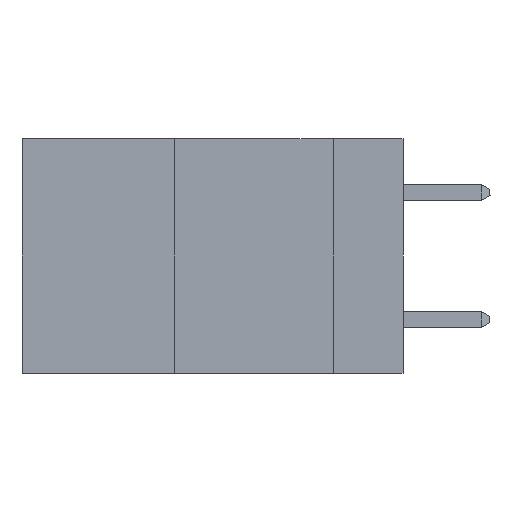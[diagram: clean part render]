
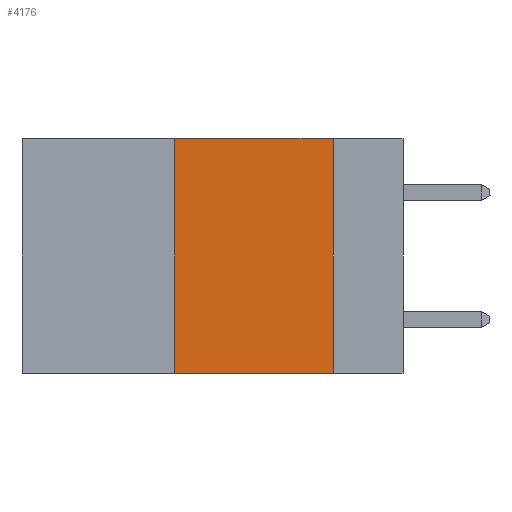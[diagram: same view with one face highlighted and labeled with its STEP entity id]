
A CAD part, left-side view. The second image highlights one B-rep face of the part: STEP entity #4176.
In plain terms, the highlighted planar face has unit normal (-1, 0, 0).
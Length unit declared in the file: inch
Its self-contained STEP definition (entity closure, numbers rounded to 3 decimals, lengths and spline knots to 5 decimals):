
#169 = CARTESIAN_POINT ( 'NONE',  ( 0., 0.36, 0. ) ) ;
#264 = DIRECTION ( 'NONE',  ( 1., 0., 0. ) ) ;
#759 = ORIENTED_EDGE ( 'NONE', *, *, #2254, .F. ) ;
#1437 = EDGE_CURVE ( 'NONE', #4268, #16691, #3382, .T. ) ;
#2254 = EDGE_CURVE ( 'NONE', #16691, #3262, #9374, .T. ) ;
#2404 = CARTESIAN_POINT ( 'NONE',  ( 0., 0.6, 0. ) ) ;
#2499 = EDGE_CURVE ( 'NONE', #23659, #3262, #10859, .T. ) ;
#2549 = ORIENTED_EDGE ( 'NONE', *, *, #15353, .F. ) ;
#2704 = ORIENTED_EDGE ( 'NONE', *, *, #1437, .F. ) ;
#3262 = VERTEX_POINT ( 'NONE', #7851 ) ;
#3382 = LINE ( 'NONE', #11134, #20433 ) ;
#3867 = LINE ( 'NONE', #169, #15531 ) ;
#4100 = CARTESIAN_POINT ( 'NONE',  ( 0., 0.11, 0. ) ) ;
#4176 = ADVANCED_FACE ( 'NONE', ( #7513 ), #15871, .F. ) ;
#4268 = VERTEX_POINT ( 'NONE', #10286 ) ;
#5139 = DIRECTION ( 'NONE',  ( 0., -1., 0. ) ) ;
#7050 = CARTESIAN_POINT ( 'NONE',  ( 0., 0.6, -0.37 ) ) ;
#7513 = FACE_OUTER_BOUND ( 'NONE', #17952, .T. ) ;
#7851 = CARTESIAN_POINT ( 'NONE',  ( 0., 0.11, -0.37 ) ) ;
#9374 = LINE ( 'NONE', #24744, #22266 ) ;
#10286 = CARTESIAN_POINT ( 'NONE',  ( 0., 0.36, 0. ) ) ;
#10859 = LINE ( 'NONE', #7050, #11379 ) ;
#11134 = CARTESIAN_POINT ( 'NONE',  ( 0., 0.6, 0. ) ) ;
#11379 = VECTOR ( 'NONE', #5139, 39.37008 ) ;
#14073 = DIRECTION ( 'NONE',  ( 0., 0., -1. ) ) ;
#15353 = EDGE_CURVE ( 'NONE', #23659, #4268, #3867, .T. ) ;
#15531 = VECTOR ( 'NONE', #17691, 39.37008 ) ;
#15871 = PLANE ( 'NONE',  #18927 ) ;
#16691 = VERTEX_POINT ( 'NONE', #4100 ) ;
#16979 = DIRECTION ( 'NONE',  ( 0., 0., -1. ) ) ;
#17377 = CARTESIAN_POINT ( 'NONE',  ( 0., 0.36, -0.37 ) ) ;
#17691 = DIRECTION ( 'NONE',  ( 0., 0., 1. ) ) ;
#17952 = EDGE_LOOP ( 'NONE', ( #759, #2704, #2549, #23083 ) ) ;
#18927 = AXIS2_PLACEMENT_3D ( 'NONE', #2404, #264, #14073 ) ;
#20433 = VECTOR ( 'NONE', #24707, 39.37008 ) ;
#22266 = VECTOR ( 'NONE', #16979, 39.37008 ) ;
#23083 = ORIENTED_EDGE ( 'NONE', *, *, #2499, .T. ) ;
#23659 = VERTEX_POINT ( 'NONE', #17377 ) ;
#24707 = DIRECTION ( 'NONE',  ( 0., -1., 0. ) ) ;
#24744 = CARTESIAN_POINT ( 'NONE',  ( 0., 0.11, 0. ) ) ;
